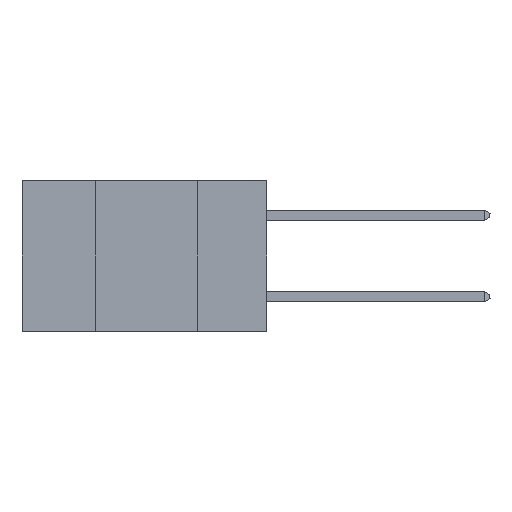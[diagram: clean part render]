
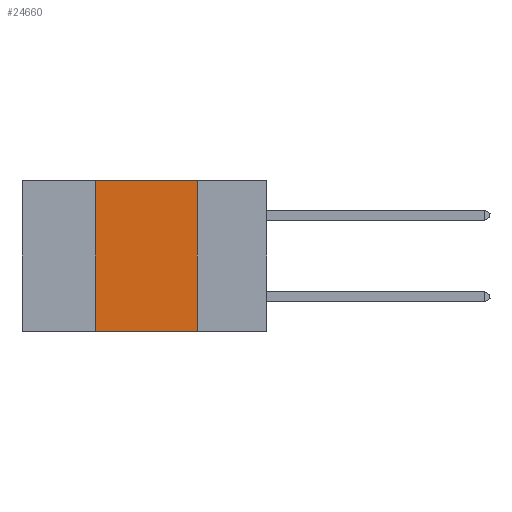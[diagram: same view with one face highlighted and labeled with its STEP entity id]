
A CAD part, left-side view. The second image highlights one B-rep face of the part: STEP entity #24660.
In plain terms, the highlighted planar face has unit normal (-1, 0, 0).
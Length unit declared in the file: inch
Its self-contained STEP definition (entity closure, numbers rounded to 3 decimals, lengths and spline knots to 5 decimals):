
#192 = AXIS2_PLACEMENT_3D ( 'NONE', #27107, #281, #15072 ) ;
#281 = DIRECTION ( 'NONE',  ( 1., 0., 0. ) ) ;
#490 = VERTEX_POINT ( 'NONE', #11711 ) ;
#552 = VECTOR ( 'NONE', #21963, 39.37008 ) ;
#2836 = CARTESIAN_POINT ( 'NONE',  ( 0., 0.17, 0. ) ) ;
#3297 = VERTEX_POINT ( 'NONE', #24449 ) ;
#4413 = CARTESIAN_POINT ( 'NONE',  ( 0., 0.42, -0.37 ) ) ;
#5117 = CARTESIAN_POINT ( 'NONE',  ( 0., 0.6, 0. ) ) ;
#5212 = DIRECTION ( 'NONE',  ( 0., -1., 0. ) ) ;
#5828 = EDGE_LOOP ( 'NONE', ( #26364, #13246, #22213, #8888 ) ) ;
#6033 = CARTESIAN_POINT ( 'NONE',  ( 0., 0.17, 0. ) ) ;
#6851 = CARTESIAN_POINT ( 'NONE',  ( 0., 0.6, -0.37 ) ) ;
#7846 = VECTOR ( 'NONE', #8753, 39.37008 ) ;
#8076 = EDGE_CURVE ( 'NONE', #19298, #490, #10714, .T. ) ;
#8578 = EDGE_CURVE ( 'NONE', #16322, #3297, #23866, .T. ) ;
#8580 = LINE ( 'NONE', #5117, #13506 ) ;
#8753 = DIRECTION ( 'NONE',  ( 0., -1., 0. ) ) ;
#8888 = ORIENTED_EDGE ( 'NONE', *, *, #13346, .T. ) ;
#10504 = PLANE ( 'NONE',  #192 ) ;
#10714 = LINE ( 'NONE', #11528, #552 ) ;
#11528 = CARTESIAN_POINT ( 'NONE',  ( 0., 0.42, 0. ) ) ;
#11711 = CARTESIAN_POINT ( 'NONE',  ( 0., 0.42, 0. ) ) ;
#11748 = VECTOR ( 'NONE', #17321, 39.37008 ) ;
#13246 = ORIENTED_EDGE ( 'NONE', *, *, #20375, .F. ) ;
#13346 = EDGE_CURVE ( 'NONE', #19298, #3297, #19007, .T. ) ;
#13506 = VECTOR ( 'NONE', #5212, 39.37008 ) ;
#15072 = DIRECTION ( 'NONE',  ( 0., 0., -1. ) ) ;
#16322 = VERTEX_POINT ( 'NONE', #6033 ) ;
#17321 = DIRECTION ( 'NONE',  ( 0., 0., -1. ) ) ;
#19007 = LINE ( 'NONE', #6851, #7846 ) ;
#19298 = VERTEX_POINT ( 'NONE', #4413 ) ;
#19911 = FACE_OUTER_BOUND ( 'NONE', #5828, .T. ) ;
#20375 = EDGE_CURVE ( 'NONE', #490, #16322, #8580, .T. ) ;
#21963 = DIRECTION ( 'NONE',  ( 0., 0., 1. ) ) ;
#22213 = ORIENTED_EDGE ( 'NONE', *, *, #8076, .F. ) ;
#23866 = LINE ( 'NONE', #2836, #11748 ) ;
#24449 = CARTESIAN_POINT ( 'NONE',  ( 0., 0.17, -0.37 ) ) ;
#24660 = ADVANCED_FACE ( 'NONE', ( #19911 ), #10504, .F. ) ;
#26364 = ORIENTED_EDGE ( 'NONE', *, *, #8578, .F. ) ;
#27107 = CARTESIAN_POINT ( 'NONE',  ( 0., 0.6, 0. ) ) ;
